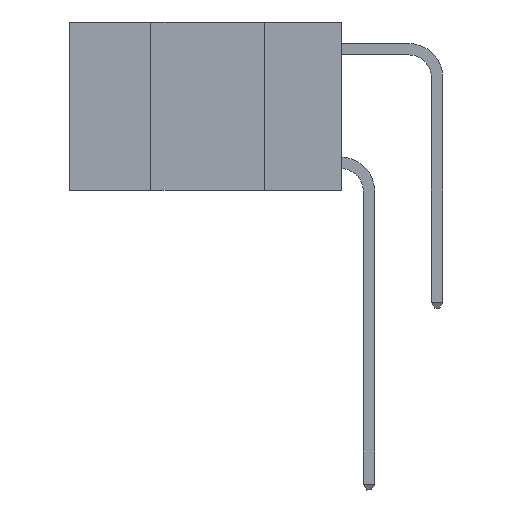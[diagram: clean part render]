
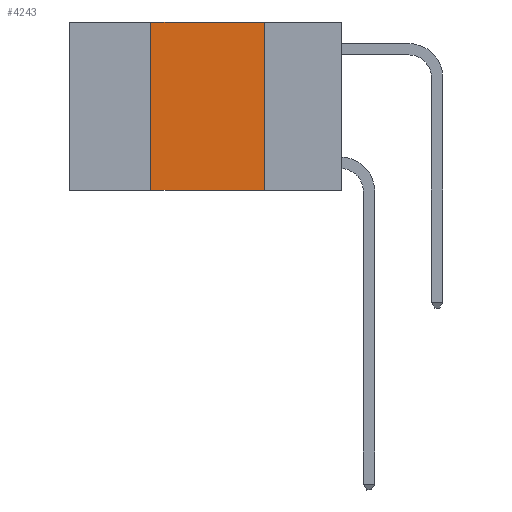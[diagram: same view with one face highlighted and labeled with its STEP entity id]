
A CAD part, left-side view. The second image highlights one B-rep face of the part: STEP entity #4243.
In plain terms, the highlighted planar face has unit normal (-1, 0, 0).
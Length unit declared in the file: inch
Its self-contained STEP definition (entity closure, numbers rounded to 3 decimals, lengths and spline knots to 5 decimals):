
#923 = FACE_OUTER_BOUND ( 'NONE', #7305, .T. ) ;
#1151 = DIRECTION ( 'NONE',  ( 0., 0., -1. ) ) ;
#1234 = VECTOR ( 'NONE', #12093, 39.37008 ) ;
#1291 = CARTESIAN_POINT ( 'NONE',  ( 0., 0.42, 0. ) ) ;
#1606 = CARTESIAN_POINT ( 'NONE',  ( 0., 0.17, 0. ) ) ;
#1833 = ORIENTED_EDGE ( 'NONE', *, *, #10146, .F. ) ;
#2246 = CARTESIAN_POINT ( 'NONE',  ( 0., 0.6, 0. ) ) ;
#2745 = ORIENTED_EDGE ( 'NONE', *, *, #9880, .T. ) ;
#3628 = LINE ( 'NONE', #1291, #1234 ) ;
#3673 = VECTOR ( 'NONE', #8373, 39.37008 ) ;
#3947 = CARTESIAN_POINT ( 'NONE',  ( 0., 0.6, -0.37 ) ) ;
#3971 = AXIS2_PLACEMENT_3D ( 'NONE', #2246, #13005, #1151 ) ;
#4243 = ADVANCED_FACE ( 'NONE', ( #923 ), #4750, .F. ) ;
#4750 = PLANE ( 'NONE',  #3971 ) ;
#4773 = CARTESIAN_POINT ( 'NONE',  ( 0., 0.17, 0. ) ) ;
#5438 = ORIENTED_EDGE ( 'NONE', *, *, #5763, .F. ) ;
#5724 = VECTOR ( 'NONE', #6344, 39.37008 ) ;
#5763 = EDGE_CURVE ( 'NONE', #7454, #12198, #8174, .T. ) ;
#5843 = CARTESIAN_POINT ( 'NONE',  ( 0., 0.6, 0. ) ) ;
#6100 = LINE ( 'NONE', #5843, #3673 ) ;
#6344 = DIRECTION ( 'NONE',  ( 0., -1., 0. ) ) ;
#6428 = VERTEX_POINT ( 'NONE', #11415 ) ;
#7305 = EDGE_LOOP ( 'NONE', ( #5438, #1833, #14779, #2745 ) ) ;
#7454 = VERTEX_POINT ( 'NONE', #4773 ) ;
#8174 = LINE ( 'NONE', #1606, #14075 ) ;
#8233 = CARTESIAN_POINT ( 'NONE',  ( 0., 0.42, 0. ) ) ;
#8373 = DIRECTION ( 'NONE',  ( 0., -1., 0. ) ) ;
#8915 = LINE ( 'NONE', #3947, #5724 ) ;
#9880 = EDGE_CURVE ( 'NONE', #6428, #12198, #8915, .T. ) ;
#10056 = CARTESIAN_POINT ( 'NONE',  ( 0., 0.17, -0.37 ) ) ;
#10146 = EDGE_CURVE ( 'NONE', #14860, #7454, #6100, .T. ) ;
#11415 = CARTESIAN_POINT ( 'NONE',  ( 0., 0.42, -0.37 ) ) ;
#11536 = EDGE_CURVE ( 'NONE', #6428, #14860, #3628, .T. ) ;
#12093 = DIRECTION ( 'NONE',  ( 0., 0., 1. ) ) ;
#12198 = VERTEX_POINT ( 'NONE', #10056 ) ;
#13005 = DIRECTION ( 'NONE',  ( 1., 0., 0. ) ) ;
#14075 = VECTOR ( 'NONE', #14825, 39.37008 ) ;
#14779 = ORIENTED_EDGE ( 'NONE', *, *, #11536, .F. ) ;
#14825 = DIRECTION ( 'NONE',  ( 0., 0., -1. ) ) ;
#14860 = VERTEX_POINT ( 'NONE', #8233 ) ;
